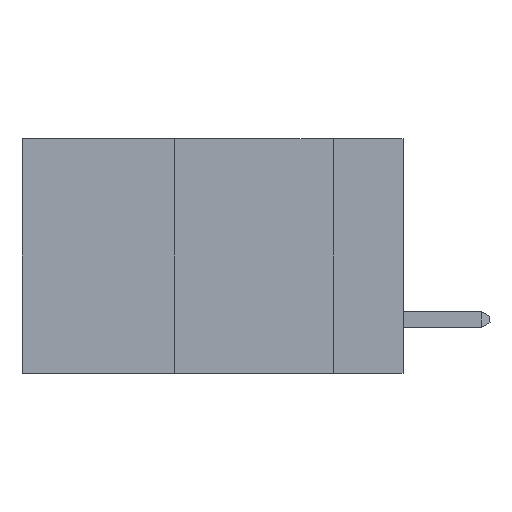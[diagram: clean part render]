
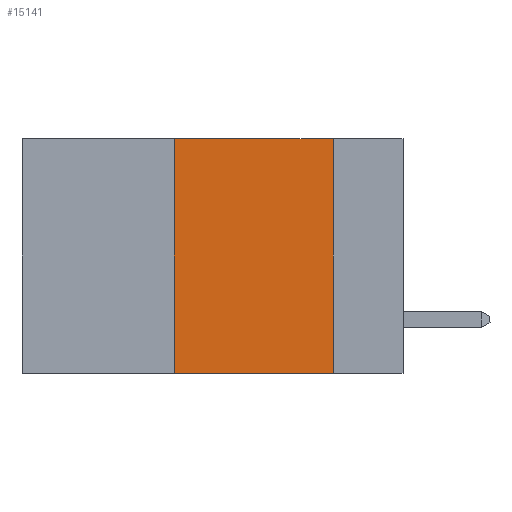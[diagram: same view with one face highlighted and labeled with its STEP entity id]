
A CAD part, left-side view. The second image highlights one B-rep face of the part: STEP entity #15141.
In plain terms, the highlighted planar face has unit normal (-1, 0, 0).
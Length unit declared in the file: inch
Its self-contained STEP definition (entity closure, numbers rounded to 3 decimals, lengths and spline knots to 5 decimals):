
#543 = CARTESIAN_POINT ( 'NONE',  ( 0., 0.36, -0.37 ) ) ;
#1093 = VERTEX_POINT ( 'NONE', #1614 ) ;
#1614 = CARTESIAN_POINT ( 'NONE',  ( 0., 0.11, -0.37 ) ) ;
#2044 = CARTESIAN_POINT ( 'NONE',  ( 0., 0.6, 0. ) ) ;
#2841 = EDGE_CURVE ( 'NONE', #3231, #23486, #15614, .T. ) ;
#3231 = VERTEX_POINT ( 'NONE', #7304 ) ;
#3320 = AXIS2_PLACEMENT_3D ( 'NONE', #21564, #9537, #23603 ) ;
#3461 = CARTESIAN_POINT ( 'NONE',  ( 0., 0.6, -0.37 ) ) ;
#5117 = FACE_OUTER_BOUND ( 'NONE', #19466, .T. ) ;
#5336 = CARTESIAN_POINT ( 'NONE',  ( 0., 0.36, 0. ) ) ;
#5533 = ORIENTED_EDGE ( 'NONE', *, *, #9991, .F. ) ;
#7304 = CARTESIAN_POINT ( 'NONE',  ( 0., 0.36, 0. ) ) ;
#7546 = DIRECTION ( 'NONE',  ( 0., -1., 0. ) ) ;
#7763 = DIRECTION ( 'NONE',  ( 0., 0., -1. ) ) ;
#7792 = EDGE_CURVE ( 'NONE', #16727, #1093, #13425, .T. ) ;
#8127 = VECTOR ( 'NONE', #7546, 39.37008 ) ;
#9537 = DIRECTION ( 'NONE',  ( 1., 0., 0. ) ) ;
#9981 = VECTOR ( 'NONE', #7763, 39.37008 ) ;
#9991 = EDGE_CURVE ( 'NONE', #16727, #3231, #24892, .T. ) ;
#12128 = DIRECTION ( 'NONE',  ( 0., -1., 0. ) ) ;
#13218 = CARTESIAN_POINT ( 'NONE',  ( 0., 0.11, 0. ) ) ;
#13425 = LINE ( 'NONE', #3461, #8127 ) ;
#15141 = ADVANCED_FACE ( 'NONE', ( #5117 ), #17418, .F. ) ;
#15614 = LINE ( 'NONE', #2044, #20204 ) ;
#16727 = VERTEX_POINT ( 'NONE', #543 ) ;
#17418 = PLANE ( 'NONE',  #3320 ) ;
#19466 = EDGE_LOOP ( 'NONE', ( #24398, #22197, #5533, #23809 ) ) ;
#20204 = VECTOR ( 'NONE', #12128, 39.37008 ) ;
#20742 = EDGE_CURVE ( 'NONE', #23486, #1093, #25391, .T. ) ;
#21564 = CARTESIAN_POINT ( 'NONE',  ( 0., 0.6, 0. ) ) ;
#21821 = CARTESIAN_POINT ( 'NONE',  ( 0., 0.11, 0. ) ) ;
#22197 = ORIENTED_EDGE ( 'NONE', *, *, #2841, .F. ) ;
#23486 = VERTEX_POINT ( 'NONE', #13218 ) ;
#23603 = DIRECTION ( 'NONE',  ( 0., 0., -1. ) ) ;
#23809 = ORIENTED_EDGE ( 'NONE', *, *, #7792, .T. ) ;
#24278 = VECTOR ( 'NONE', #25404, 39.37008 ) ;
#24398 = ORIENTED_EDGE ( 'NONE', *, *, #20742, .F. ) ;
#24892 = LINE ( 'NONE', #5336, #24278 ) ;
#25391 = LINE ( 'NONE', #21821, #9981 ) ;
#25404 = DIRECTION ( 'NONE',  ( 0., 0., 1. ) ) ;
